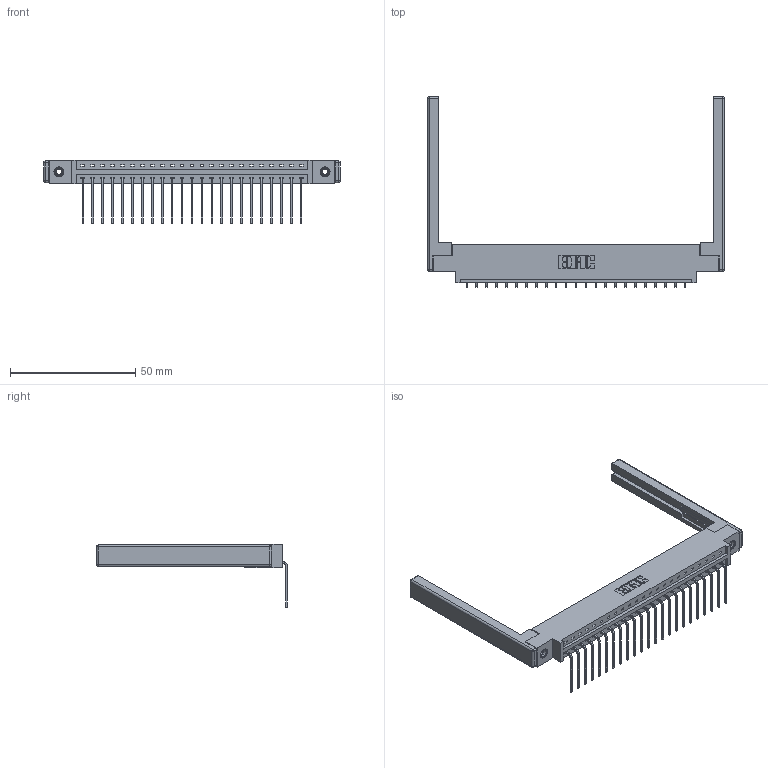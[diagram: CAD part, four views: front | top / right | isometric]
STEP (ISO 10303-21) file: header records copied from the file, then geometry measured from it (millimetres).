
FILE_DESCRIPTION (( 'STEP AP203' ), '1' );
FILE_NAME ('387-023-559-668.STEP', '2019-10-03T03:39:27', ( '' ), ( '' ), 'SwSTEP 2.0', 'SolidWorks 2016', '' );
FILE_SCHEMA (( 'CONFIG_CONTROL_DESIGN' ));
Length unit declared in the file: inch
Products named in the file (5): 387-023-559-668; 345-250-001_345-250-001-102; 345-292-001_558 559 Tail - 1; 337 Part_0.170 Offset - 0.156 Dia-TI; 307-220-068
Assembly tree (28 placements, depth 2):
  387-023-559-668
    337 Part_0.170 Offset - 0.156 Dia-TI
    345-292-001_558 559 Tail - 1  x23
    345-250-001_345-250-001-102  x2
    307-220-068  x2
Bounding box: 118.57 x 76.14 x 25.53 mm (x, y, z)
Volume: 16435.7 mm3; surface area: 17000.6 mm2
Topology: 28 solids, 28 shells, 1744 faces, 5175 edges, 3398 vertices
Faces by surface type: plane 1266, cylinder 454, cone 12, sphere 8, torus 4
Entity records: 22530 total; most frequent: CARTESIAN_POINT 3880, ORIENTED_EDGE 3828, DIRECTION 3378, EDGE_CURVE 1914, VECTOR 1736, LINE 1736, VERTEX_POINT 1266, AXIS2_PLACEMENT_3D 821
